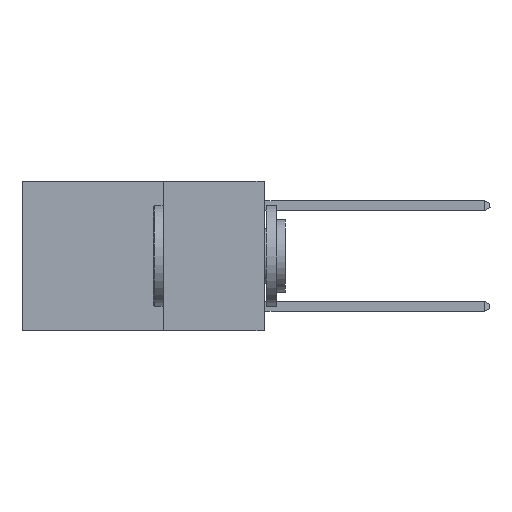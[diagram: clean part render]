
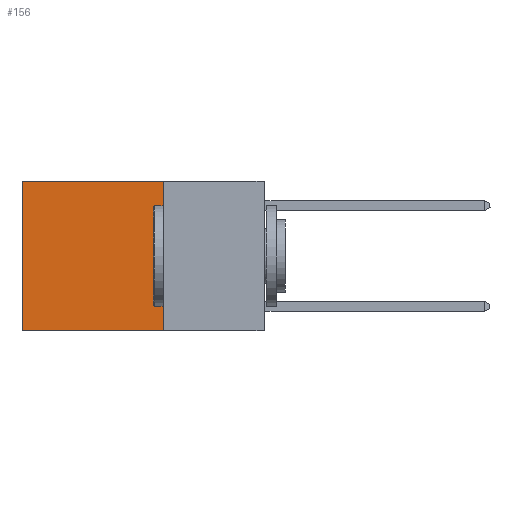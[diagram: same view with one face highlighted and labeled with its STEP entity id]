
A CAD part, left-side view. The second image highlights one B-rep face of the part: STEP entity #156.
In plain terms, the highlighted planar face has unit normal (-1, 0, 0).
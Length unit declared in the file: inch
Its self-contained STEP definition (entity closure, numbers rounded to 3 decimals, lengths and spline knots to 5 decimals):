
#127 = CARTESIAN_POINT ( 'NONE',  ( 0.2625, 0.25, 0. ) ) ;
#156 = ADVANCED_FACE ( 'NONE', ( #17062 ), #7777, .F. ) ;
#157 = VERTEX_POINT ( 'NONE', #7682 ) ;
#362 = EDGE_CURVE ( 'NONE', #2694, #12330, #14912, .T. ) ;
#413 = CARTESIAN_POINT ( 'NONE',  ( 0.2625, 0.25, 0. ) ) ;
#597 = DIRECTION ( 'NONE',  ( 0., 0., -1. ) ) ;
#670 = CARTESIAN_POINT ( 'NONE',  ( 0.2625, 0.6, 0. ) ) ;
#1005 = DIRECTION ( 'NONE',  ( 0., 0., -1. ) ) ;
#1317 = ORIENTED_EDGE ( 'NONE', *, *, #2688, .T. ) ;
#2577 = DIRECTION ( 'NONE',  ( 0., 1., 0. ) ) ;
#2688 = EDGE_CURVE ( 'NONE', #13965, #157, #8087, .T. ) ;
#2694 = VERTEX_POINT ( 'NONE', #4165 ) ;
#2908 = EDGE_CURVE ( 'NONE', #157, #12330, #10309, .T. ) ;
#3009 = AXIS2_PLACEMENT_3D ( 'NONE', #9210, #14727, #1005 ) ;
#4108 = EDGE_CURVE ( 'NONE', #13965, #2694, #13885, .T. ) ;
#4165 = CARTESIAN_POINT ( 'NONE',  ( 0.2625, 0.25, -0.37 ) ) ;
#4779 = DIRECTION ( 'NONE',  ( 0., 0., -1. ) ) ;
#6800 = CARTESIAN_POINT ( 'NONE',  ( 0.2625, 0.25, -0.37 ) ) ;
#6916 = VECTOR ( 'NONE', #2577, 39.37008 ) ;
#6961 = CARTESIAN_POINT ( 'NONE',  ( 0.2625, 0.25, 0. ) ) ;
#7682 = CARTESIAN_POINT ( 'NONE',  ( 0.2625, 0.6, 0. ) ) ;
#7777 = PLANE ( 'NONE',  #3009 ) ;
#8087 = LINE ( 'NONE', #127, #6916 ) ;
#8835 = ORIENTED_EDGE ( 'NONE', *, *, #362, .F. ) ;
#9210 = CARTESIAN_POINT ( 'NONE',  ( 0.2625, 0.25, 0. ) ) ;
#9563 = DIRECTION ( 'NONE',  ( 0., 1., 0. ) ) ;
#9837 = CARTESIAN_POINT ( 'NONE',  ( 0.2625, 0.6, -0.37 ) ) ;
#10309 = LINE ( 'NONE', #670, #11585 ) ;
#10511 = EDGE_LOOP ( 'NONE', ( #14481, #8835, #17452, #1317 ) ) ;
#11585 = VECTOR ( 'NONE', #4779, 39.37008 ) ;
#12330 = VERTEX_POINT ( 'NONE', #9837 ) ;
#13885 = LINE ( 'NONE', #413, #14533 ) ;
#13965 = VERTEX_POINT ( 'NONE', #6961 ) ;
#14481 = ORIENTED_EDGE ( 'NONE', *, *, #2908, .T. ) ;
#14533 = VECTOR ( 'NONE', #597, 39.37008 ) ;
#14727 = DIRECTION ( 'NONE',  ( 1., 0., 0. ) ) ;
#14912 = LINE ( 'NONE', #6800, #15611 ) ;
#15611 = VECTOR ( 'NONE', #9563, 39.37008 ) ;
#17062 = FACE_OUTER_BOUND ( 'NONE', #10511, .T. ) ;
#17452 = ORIENTED_EDGE ( 'NONE', *, *, #4108, .F. ) ;
